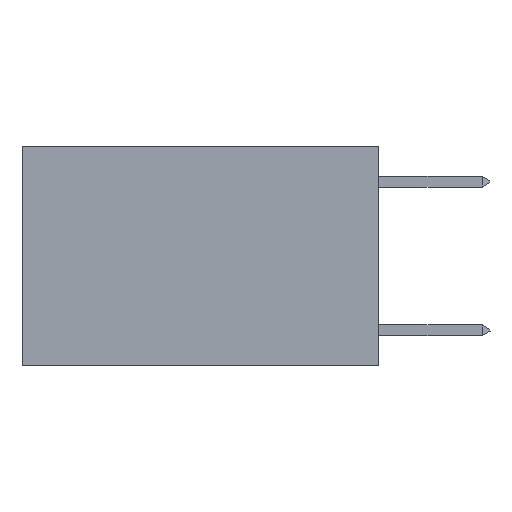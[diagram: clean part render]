
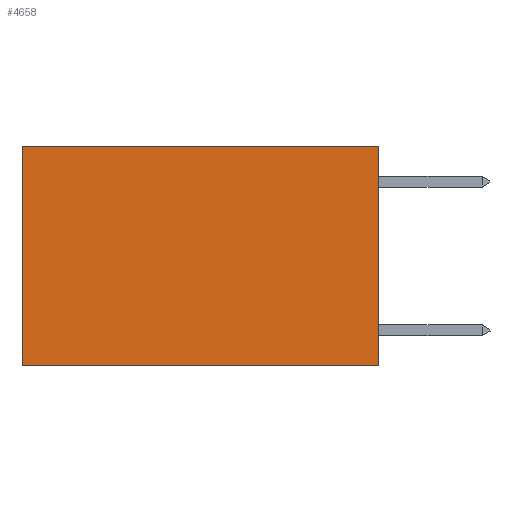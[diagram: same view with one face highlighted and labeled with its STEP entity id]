
A CAD part, left-side view. The second image highlights one B-rep face of the part: STEP entity #4658.
In plain terms, the highlighted planar face has unit normal (-1, 0, 0).
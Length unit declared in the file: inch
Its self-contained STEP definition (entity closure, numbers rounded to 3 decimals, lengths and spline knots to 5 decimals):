
#59 = VECTOR ( 'NONE', #5070, 39.37008 ) ;
#294 = ORIENTED_EDGE ( 'NONE', *, *, #2800, .T. ) ;
#448 = ORIENTED_EDGE ( 'NONE', *, *, #6196, .F. ) ;
#735 = CARTESIAN_POINT ( 'NONE',  ( 0.2625, 0.6, 0. ) ) ;
#1176 = AXIS2_PLACEMENT_3D ( 'NONE', #1295, #7510, #3395 ) ;
#1295 = CARTESIAN_POINT ( 'NONE',  ( 0.2625, 0., 0. ) ) ;
#1702 = LINE ( 'NONE', #7068, #8797 ) ;
#2217 = FACE_OUTER_BOUND ( 'NONE', #3488, .T. ) ;
#2434 = EDGE_CURVE ( 'NONE', #8724, #3580, #1702, .T. ) ;
#2800 = EDGE_CURVE ( 'NONE', #8724, #8083, #3346, .T. ) ;
#2828 = DIRECTION ( 'NONE',  ( 0., 0., -1. ) ) ;
#3140 = VECTOR ( 'NONE', #5768, 39.37008 ) ;
#3346 = LINE ( 'NONE', #4774, #3140 ) ;
#3395 = DIRECTION ( 'NONE',  ( 0., 0., -1. ) ) ;
#3488 = EDGE_LOOP ( 'NONE', ( #4555, #448, #5189, #294 ) ) ;
#3580 = VERTEX_POINT ( 'NONE', #4524 ) ;
#3608 = VECTOR ( 'NONE', #4964, 39.37008 ) ;
#3652 = CARTESIAN_POINT ( 'NONE',  ( 0.2625, 0.6, 0. ) ) ;
#3653 = CARTESIAN_POINT ( 'NONE',  ( 0.2625, 0., -0.37 ) ) ;
#4524 = CARTESIAN_POINT ( 'NONE',  ( 0.2625, 0., -0.37 ) ) ;
#4555 = ORIENTED_EDGE ( 'NONE', *, *, #7989, .T. ) ;
#4658 = ADVANCED_FACE ( 'NONE', ( #2217 ), #8165, .F. ) ;
#4774 = CARTESIAN_POINT ( 'NONE',  ( 0.2625, 0., 0. ) ) ;
#4964 = DIRECTION ( 'NONE',  ( 0., 0., -1. ) ) ;
#5070 = DIRECTION ( 'NONE',  ( 0., 1., 0. ) ) ;
#5189 = ORIENTED_EDGE ( 'NONE', *, *, #2434, .F. ) ;
#5472 = LINE ( 'NONE', #3653, #59 ) ;
#5768 = DIRECTION ( 'NONE',  ( 0., 1., 0. ) ) ;
#6196 = EDGE_CURVE ( 'NONE', #3580, #8113, #5472, .T. ) ;
#7026 = LINE ( 'NONE', #735, #3608 ) ;
#7068 = CARTESIAN_POINT ( 'NONE',  ( 0.2625, 0., 0. ) ) ;
#7510 = DIRECTION ( 'NONE',  ( 1., 0., 0. ) ) ;
#7989 = EDGE_CURVE ( 'NONE', #8083, #8113, #7026, .T. ) ;
#8083 = VERTEX_POINT ( 'NONE', #3652 ) ;
#8113 = VERTEX_POINT ( 'NONE', #8470 ) ;
#8165 = PLANE ( 'NONE',  #1176 ) ;
#8457 = CARTESIAN_POINT ( 'NONE',  ( 0.2625, 0., 0. ) ) ;
#8470 = CARTESIAN_POINT ( 'NONE',  ( 0.2625, 0.6, -0.37 ) ) ;
#8724 = VERTEX_POINT ( 'NONE', #8457 ) ;
#8797 = VECTOR ( 'NONE', #2828, 39.37008 ) ;
